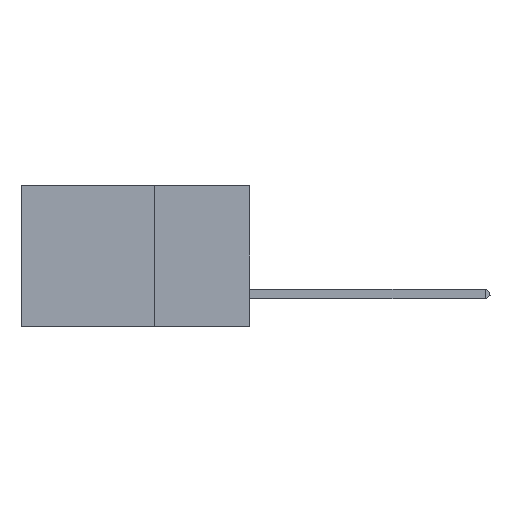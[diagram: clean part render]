
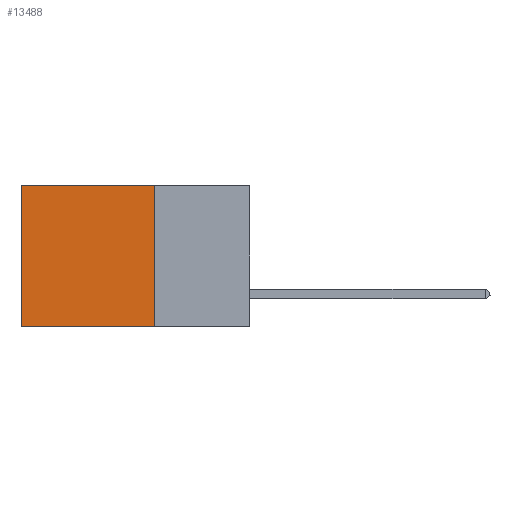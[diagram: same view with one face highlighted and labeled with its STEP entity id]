
A CAD part, left-side view. The second image highlights one B-rep face of the part: STEP entity #13488.
In plain terms, the highlighted planar face has unit normal (-1, 0, 0).
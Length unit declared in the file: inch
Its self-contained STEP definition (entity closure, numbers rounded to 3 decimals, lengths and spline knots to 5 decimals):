
#1455 = VECTOR ( 'NONE', #15084, 39.37008 ) ;
#3305 = VERTEX_POINT ( 'NONE', #16254 ) ;
#4024 = CARTESIAN_POINT ( 'NONE',  ( 0.2875, 0.25, -0.37 ) ) ;
#7060 = DIRECTION ( 'NONE',  ( 0., 1., 0. ) ) ;
#10242 = CARTESIAN_POINT ( 'NONE',  ( 0.2875, 0.6, -0.37 ) ) ;
#12019 = CARTESIAN_POINT ( 'NONE',  ( 0.2875, 0.25, 0. ) ) ;
#13488 = ADVANCED_FACE ( 'NONE', ( #25988 ), #25212, .F. ) ;
#14434 = EDGE_CURVE ( 'NONE', #29053, #24864, #36458, .T. ) ;
#14771 = DIRECTION ( 'NONE',  ( 0., 0., -1. ) ) ;
#15084 = DIRECTION ( 'NONE',  ( 0., 1., 0. ) ) ;
#15295 = ORIENTED_EDGE ( 'NONE', *, *, #32535, .T. ) ;
#15323 = CARTESIAN_POINT ( 'NONE',  ( 0.2875, 0.25, 0. ) ) ;
#16003 = ORIENTED_EDGE ( 'NONE', *, *, #29582, .F. ) ;
#16254 = CARTESIAN_POINT ( 'NONE',  ( 0.2875, 0.25, -0.37 ) ) ;
#16630 = VERTEX_POINT ( 'NONE', #10242 ) ;
#17327 = DIRECTION ( 'NONE',  ( 0., 0., -1. ) ) ;
#22242 = DIRECTION ( 'NONE',  ( 0., 0., -1. ) ) ;
#22620 = ORIENTED_EDGE ( 'NONE', *, *, #14434, .T. ) ;
#23221 = AXIS2_PLACEMENT_3D ( 'NONE', #27982, #33989, #22242 ) ;
#24361 = EDGE_LOOP ( 'NONE', ( #15295, #16003, #35257, #22620 ) ) ;
#24864 = VERTEX_POINT ( 'NONE', #27474 ) ;
#25212 = PLANE ( 'NONE',  #23221 ) ;
#25280 = VECTOR ( 'NONE', #17327, 39.37008 ) ;
#25288 = VECTOR ( 'NONE', #14771, 39.37008 ) ;
#25988 = FACE_OUTER_BOUND ( 'NONE', #24361, .T. ) ;
#27474 = CARTESIAN_POINT ( 'NONE',  ( 0.2875, 0.6, 0. ) ) ;
#27519 = CARTESIAN_POINT ( 'NONE',  ( 0.2875, 0.25, 0. ) ) ;
#27982 = CARTESIAN_POINT ( 'NONE',  ( 0.2875, 0.25, 0. ) ) ;
#27995 = VECTOR ( 'NONE', #7060, 39.37008 ) ;
#29053 = VERTEX_POINT ( 'NONE', #27519 ) ;
#29582 = EDGE_CURVE ( 'NONE', #3305, #16630, #35607, .T. ) ;
#32026 = LINE ( 'NONE', #12019, #25288 ) ;
#32535 = EDGE_CURVE ( 'NONE', #24864, #16630, #36511, .T. ) ;
#33989 = DIRECTION ( 'NONE',  ( 1., 0., 0. ) ) ;
#35011 = CARTESIAN_POINT ( 'NONE',  ( 0.2875, 0.6, 0. ) ) ;
#35257 = ORIENTED_EDGE ( 'NONE', *, *, #36964, .F. ) ;
#35607 = LINE ( 'NONE', #4024, #27995 ) ;
#36458 = LINE ( 'NONE', #15323, #1455 ) ;
#36511 = LINE ( 'NONE', #35011, #25280 ) ;
#36964 = EDGE_CURVE ( 'NONE', #29053, #3305, #32026, .T. ) ;
